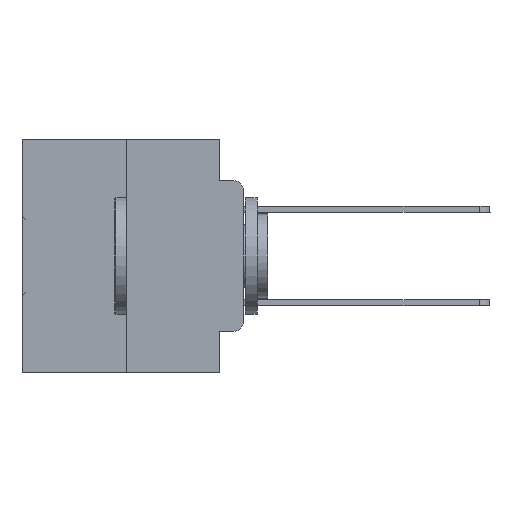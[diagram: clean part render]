
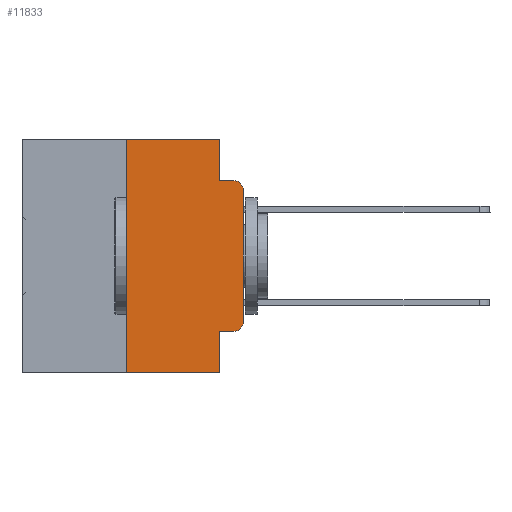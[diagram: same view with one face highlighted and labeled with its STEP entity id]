
A CAD part, left-side view. The second image highlights one B-rep face of the part: STEP entity #11833.
In plain terms, the highlighted planar face has unit normal (-1, 0, 0).
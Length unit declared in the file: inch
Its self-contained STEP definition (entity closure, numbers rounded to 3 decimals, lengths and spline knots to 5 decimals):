
#403 = EDGE_CURVE ( 'NONE', #21722, #6422, #7725, .T. ) ;
#899 = VERTEX_POINT ( 'NONE', #19069 ) ;
#1243 = VECTOR ( 'NONE', #30856, 39.37008 ) ;
#1358 = CARTESIAN_POINT ( 'NONE',  ( 0., 0., -0.3915 ) ) ;
#1754 = VECTOR ( 'NONE', #15301, 39.37008 ) ;
#2682 = CARTESIAN_POINT ( 'NONE',  ( 0., 0.051, -0.4115 ) ) ;
#3191 = DIRECTION ( 'NONE',  ( 0., 0., -1. ) ) ;
#3247 = ORIENTED_EDGE ( 'NONE', *, *, #6789, .T. ) ;
#3438 = ORIENTED_EDGE ( 'NONE', *, *, #34416, .T. ) ;
#3733 = LINE ( 'NONE', #24218, #17416 ) ;
#3783 = ORIENTED_EDGE ( 'NONE', *, *, #29592, .F. ) ;
#3863 = CARTESIAN_POINT ( 'NONE',  ( 0., 0.473, -0.5 ) ) ;
#4175 = DIRECTION ( 'NONE',  ( 0., 0., 1. ) ) ;
#4317 = VECTOR ( 'NONE', #4175, 39.37008 ) ;
#4580 = EDGE_CURVE ( 'NONE', #6109, #18623, #5483, .T. ) ;
#5118 = DIRECTION ( 'NONE',  ( 0., 0., -1. ) ) ;
#5228 = CARTESIAN_POINT ( 'NONE',  ( 0., 0.02, -0.4115 ) ) ;
#5276 = CARTESIAN_POINT ( 'NONE',  ( 0., 0.25, 0. ) ) ;
#5483 = LINE ( 'NONE', #32458, #33573 ) ;
#5598 = CARTESIAN_POINT ( 'NONE',  ( 0., 0.473, 0. ) ) ;
#5638 = VECTOR ( 'NONE', #29725, 39.37008 ) ;
#6109 = VERTEX_POINT ( 'NONE', #2682 ) ;
#6110 = EDGE_CURVE ( 'NONE', #13527, #23659, #14792, .T. ) ;
#6422 = VERTEX_POINT ( 'NONE', #11693 ) ;
#6789 = EDGE_CURVE ( 'NONE', #23659, #899, #30112, .T. ) ;
#6932 = DIRECTION ( 'NONE',  ( 0., 0., 1. ) ) ;
#7294 = ORIENTED_EDGE ( 'NONE', *, *, #13754, .F. ) ;
#7505 = VECTOR ( 'NONE', #6932, 39.37008 ) ;
#7725 = LINE ( 'NONE', #3863, #1243 ) ;
#8650 = EDGE_LOOP ( 'NONE', ( #13514, #3247, #33888, #21262, #3783, #31943, #26494, #7294, #16284, #3438 ) ) ;
#9170 = EDGE_CURVE ( 'NONE', #35033, #33314, #32876, .T. ) ;
#9456 = DIRECTION ( 'NONE',  ( -1., 0., 0. ) ) ;
#9785 = AXIS2_PLACEMENT_3D ( 'NONE', #23716, #26697, #10347 ) ;
#10347 = DIRECTION ( 'NONE',  ( 0., 0., -1. ) ) ;
#11116 = PLANE ( 'NONE',  #22717 ) ;
#11204 = VECTOR ( 'NONE', #3191, 39.37008 ) ;
#11561 = CARTESIAN_POINT ( 'NONE',  ( 0., 0.25, -0.5 ) ) ;
#11693 = CARTESIAN_POINT ( 'NONE',  ( 0., 0.051, -0.5 ) ) ;
#11833 = ADVANCED_FACE ( 'NONE', ( #35285 ), #11116, .F. ) ;
#13514 = ORIENTED_EDGE ( 'NONE', *, *, #6110, .T. ) ;
#13527 = VERTEX_POINT ( 'NONE', #1358 ) ;
#13754 = EDGE_CURVE ( 'NONE', #6109, #6422, #3733, .T. ) ;
#13860 = DIRECTION ( 'NONE',  ( 1., 0., 0. ) ) ;
#13978 = CARTESIAN_POINT ( 'NONE',  ( 0., 0., 0. ) ) ;
#14792 = LINE ( 'NONE', #13978, #7505 ) ;
#15012 = CARTESIAN_POINT ( 'NONE',  ( 0., 0., -0.1085 ) ) ;
#15301 = DIRECTION ( 'NONE',  ( 0., -1., 0. ) ) ;
#15752 = CARTESIAN_POINT ( 'NONE',  ( 0., 0.051, -0.0885 ) ) ;
#16284 = ORIENTED_EDGE ( 'NONE', *, *, #4580, .T. ) ;
#16735 = EDGE_CURVE ( 'NONE', #21722, #19884, #33269, .T. ) ;
#16869 = AXIS2_PLACEMENT_3D ( 'NONE', #25812, #9456, #28526 ) ;
#17201 = LINE ( 'NONE', #34267, #1754 ) ;
#17416 = VECTOR ( 'NONE', #5118, 39.37008 ) ;
#18623 = VERTEX_POINT ( 'NONE', #5228 ) ;
#19069 = CARTESIAN_POINT ( 'NONE',  ( 0., 0.02, -0.0885 ) ) ;
#19884 = VERTEX_POINT ( 'NONE', #5276 ) ;
#20217 = EDGE_CURVE ( 'NONE', #33314, #899, #27410, .T. ) ;
#21262 = ORIENTED_EDGE ( 'NONE', *, *, #9170, .F. ) ;
#21722 = VERTEX_POINT ( 'NONE', #11561 ) ;
#22717 = AXIS2_PLACEMENT_3D ( 'NONE', #5598, #13860, #32840 ) ;
#23659 = VERTEX_POINT ( 'NONE', #15012 ) ;
#23716 = CARTESIAN_POINT ( 'NONE',  ( 0., 0.02, -0.1085 ) ) ;
#24218 = CARTESIAN_POINT ( 'NONE',  ( 0., 0.051, 0. ) ) ;
#25028 = CARTESIAN_POINT ( 'NONE',  ( 0., 0.051, 0. ) ) ;
#25812 = CARTESIAN_POINT ( 'NONE',  ( 0., 0.02, -0.3915 ) ) ;
#26027 = CARTESIAN_POINT ( 'NONE',  ( 0., 0.25, 0. ) ) ;
#26494 = ORIENTED_EDGE ( 'NONE', *, *, #403, .T. ) ;
#26697 = DIRECTION ( 'NONE',  ( -1., 0., 0. ) ) ;
#27020 = CARTESIAN_POINT ( 'NONE',  ( 0., 0.051, -0.0885 ) ) ;
#27410 = LINE ( 'NONE', #27020, #5638 ) ;
#28526 = DIRECTION ( 'NONE',  ( 0., 0., -1. ) ) ;
#29592 = EDGE_CURVE ( 'NONE', #19884, #35033, #17201, .T. ) ;
#29725 = DIRECTION ( 'NONE',  ( 0., -1., 0. ) ) ;
#30112 = CIRCLE ( 'NONE', #9785, 0.02 ) ;
#30856 = DIRECTION ( 'NONE',  ( 0., -1., 0. ) ) ;
#31943 = ORIENTED_EDGE ( 'NONE', *, *, #16735, .F. ) ;
#32458 = CARTESIAN_POINT ( 'NONE',  ( 0., 0.051, -0.4115 ) ) ;
#32840 = DIRECTION ( 'NONE',  ( 0., 0., -1. ) ) ;
#32876 = LINE ( 'NONE', #25028, #11204 ) ;
#33269 = LINE ( 'NONE', #26027, #4317 ) ;
#33314 = VERTEX_POINT ( 'NONE', #15752 ) ;
#33553 = CARTESIAN_POINT ( 'NONE',  ( 0., 0.051, 0. ) ) ;
#33573 = VECTOR ( 'NONE', #35143, 39.37008 ) ;
#33795 = CIRCLE ( 'NONE', #16869, 0.02 ) ;
#33888 = ORIENTED_EDGE ( 'NONE', *, *, #20217, .F. ) ;
#34267 = CARTESIAN_POINT ( 'NONE',  ( 0., 0.473, 0. ) ) ;
#34416 = EDGE_CURVE ( 'NONE', #18623, #13527, #33795, .T. ) ;
#35033 = VERTEX_POINT ( 'NONE', #33553 ) ;
#35143 = DIRECTION ( 'NONE',  ( 0., -1., 0. ) ) ;
#35285 = FACE_OUTER_BOUND ( 'NONE', #8650, .T. ) ;
